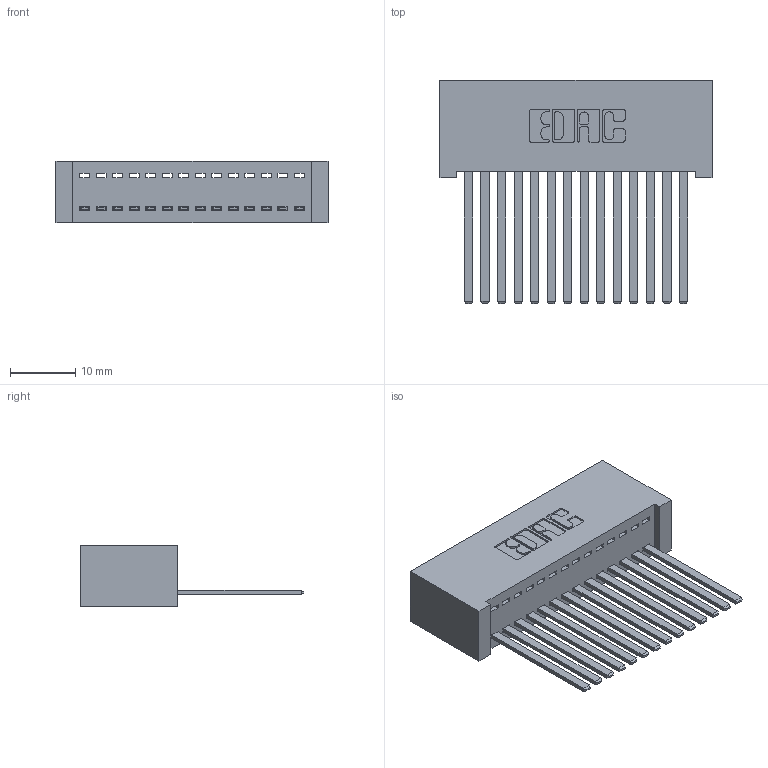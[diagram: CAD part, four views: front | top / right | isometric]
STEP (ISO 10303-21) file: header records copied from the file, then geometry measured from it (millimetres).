
FILE_DESCRIPTION (( 'STEP AP203' ), '1' );
FILE_NAME ('342-014-544-101.STEP', '2019-10-01T17:58:48', ( '' ), ( '' ), 'SwSTEP 2.0', 'SolidWorks 2016', '' );
FILE_SCHEMA (( 'CONFIG_CONTROL_DESIGN' ));
Length unit declared in the file: inch
Products named in the file (3): 342-014-544-101; 342 Part_Lugless; 345-292-001_345-293-144
Assembly tree (15 placements, depth 2):
  342-014-544-101
    342 Part_Lugless
    345-292-001_345-293-144  x14
Bounding box: 41.81 x 34.3 x 9.4 mm (x, y, z)
Volume: 4133.7 mm3; surface area: 6332.2 mm2
Topology: 15 solids, 15 shells, 830 faces, 2487 edges, 1638 vertices
Faces by surface type: plane 594, cylinder 236
Entity records: 11587 total; most frequent: CARTESIAN_POINT 2008, ORIENTED_EDGE 1958, DIRECTION 1739, EDGE_CURVE 979, VECTOR 863, LINE 863, VERTEX_POINT 650, AXIS2_PLACEMENT_3D 438
